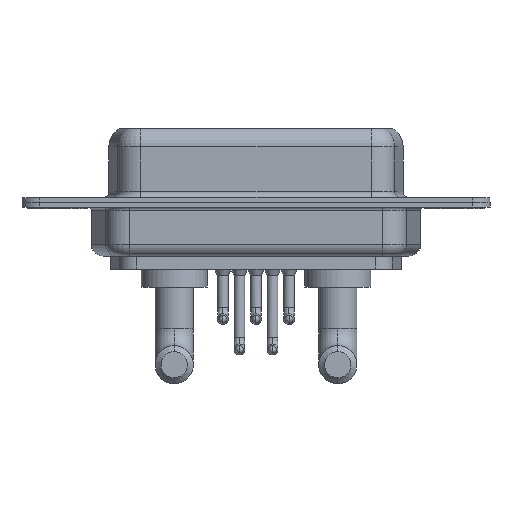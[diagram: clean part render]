
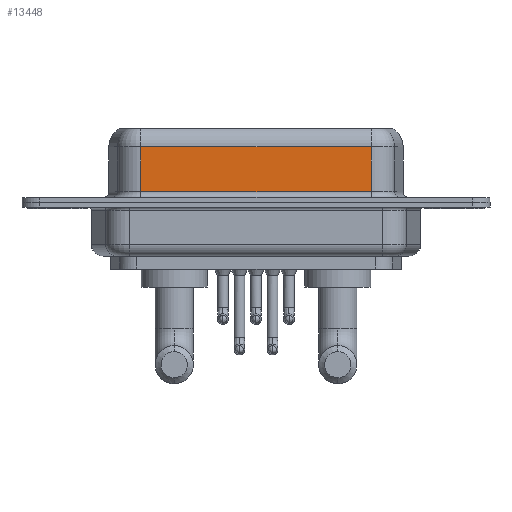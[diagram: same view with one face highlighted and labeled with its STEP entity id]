
A CAD part, front view. The second image highlights one B-rep face of the part: STEP entity #13448.
In plain terms, the highlighted planar face has unit normal (0, -1, 0).
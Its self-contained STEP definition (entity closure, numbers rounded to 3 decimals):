
#206 = VERTEX_POINT ( 'NONE', #14656 ) ;
#300 = EDGE_CURVE ( 'NONE', #1941, #206, #8706, .T. ) ;
#522 = CARTESIAN_POINT ( 'NONE',  ( 26.287, -3.95, 4.65 ) ) ;
#1896 = VECTOR ( 'NONE', #13835, 1000. ) ;
#1941 = VERTEX_POINT ( 'NONE', #9138 ) ;
#2499 = ORIENTED_EDGE ( 'NONE', *, *, #8184, .T. ) ;
#3974 = VECTOR ( 'NONE', #11278, 1000. ) ;
#4523 = EDGE_CURVE ( 'NONE', #5213, #1941, #13121, .T. ) ;
#5213 = VERTEX_POINT ( 'NONE', #13829 ) ;
#5644 = CARTESIAN_POINT ( 'NONE',  ( 26.287, -3.95, 6.4 ) ) ;
#6000 = EDGE_CURVE ( 'NONE', #5213, #14529, #10077, .T. ) ;
#6797 = CARTESIAN_POINT ( 'NONE',  ( 26.287, -3.95, 6.4 ) ) ;
#6957 = VECTOR ( 'NONE', #10917, 1000. ) ;
#7934 = FACE_OUTER_BOUND ( 'NONE', #9463, .T. ) ;
#8117 = CARTESIAN_POINT ( 'NONE',  ( 26.287, -3.95, 0.9 ) ) ;
#8184 = EDGE_CURVE ( 'NONE', #206, #14529, #15051, .T. ) ;
#8237 = DIRECTION ( 'NONE',  ( 0., 0., 1. ) ) ;
#8563 = DIRECTION ( 'NONE',  ( 0., 0., -1. ) ) ;
#8706 = LINE ( 'NONE', #9867, #13527 ) ;
#9138 = CARTESIAN_POINT ( 'NONE',  ( 7.013, -3.95, 4.65 ) ) ;
#9463 = EDGE_LOOP ( 'NONE', ( #9723, #13784, #13443, #2499 ) ) ;
#9723 = ORIENTED_EDGE ( 'NONE', *, *, #6000, .F. ) ;
#9867 = CARTESIAN_POINT ( 'NONE',  ( 7.013, -3.95, 6.4 ) ) ;
#9955 = CARTESIAN_POINT ( 'NONE',  ( 26.287, -3.95, 0.9 ) ) ;
#10077 = LINE ( 'NONE', #5644, #3974 ) ;
#10917 = DIRECTION ( 'NONE',  ( -1., 0., 0. ) ) ;
#11278 = DIRECTION ( 'NONE',  ( 0., 0., -1. ) ) ;
#11425 = DIRECTION ( 'NONE',  ( 0., 1., 0. ) ) ;
#11481 = AXIS2_PLACEMENT_3D ( 'NONE', #6797, #11425, #8237 ) ;
#12574 = PLANE ( 'NONE',  #11481 ) ;
#13121 = LINE ( 'NONE', #522, #6957 ) ;
#13443 = ORIENTED_EDGE ( 'NONE', *, *, #300, .T. ) ;
#13448 = ADVANCED_FACE ( 'NONE', ( #7934 ), #12574, .F. ) ;
#13527 = VECTOR ( 'NONE', #8563, 1000. ) ;
#13784 = ORIENTED_EDGE ( 'NONE', *, *, #4523, .T. ) ;
#13829 = CARTESIAN_POINT ( 'NONE',  ( 26.287, -3.95, 4.65 ) ) ;
#13835 = DIRECTION ( 'NONE',  ( 1., 0., 0. ) ) ;
#14529 = VERTEX_POINT ( 'NONE', #9955 ) ;
#14656 = CARTESIAN_POINT ( 'NONE',  ( 7.013, -3.95, 0.9 ) ) ;
#15051 = LINE ( 'NONE', #8117, #1896 ) ;
